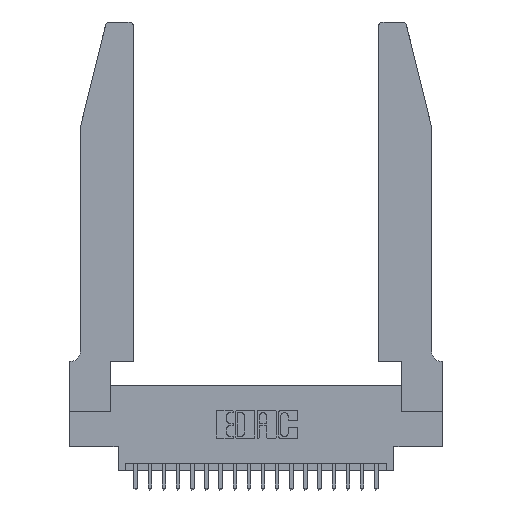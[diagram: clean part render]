
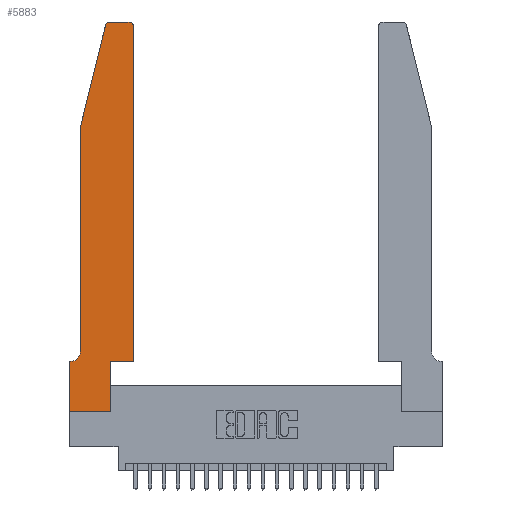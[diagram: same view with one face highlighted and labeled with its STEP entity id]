
A CAD part, top view. The second image highlights one B-rep face of the part: STEP entity #5883.
In plain terms, the highlighted planar face has unit normal (0, 0, 1).
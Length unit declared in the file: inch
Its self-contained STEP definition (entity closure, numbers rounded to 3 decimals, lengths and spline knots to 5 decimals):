
#41 = CARTESIAN_POINT ( 'NONE',  ( 0., 0., 0.37 ) ) ;
#44 = EDGE_CURVE ( 'NONE', #14610, #19202, #10375, .T. ) ;
#132 = AXIS2_PLACEMENT_3D ( 'NONE', #1566, #18614, #13588 ) ;
#656 = ORIENTED_EDGE ( 'NONE', *, *, #984, .T. ) ;
#933 = VERTEX_POINT ( 'NONE', #8329 ) ;
#984 = EDGE_CURVE ( 'NONE', #8225, #11975, #17523, .T. ) ;
#1009 = ORIENTED_EDGE ( 'NONE', *, *, #20802, .T. ) ;
#1018 = CARTESIAN_POINT ( 'NONE',  ( 0.4205, 2.72, 0.37 ) ) ;
#1566 = CARTESIAN_POINT ( 'NONE',  ( 0.0055, 0.42, 0.37 ) ) ;
#1724 = CARTESIAN_POINT ( 'NONE',  ( 0., 0.35, 0.37 ) ) ;
#2267 = CARTESIAN_POINT ( 'NONE',  ( 0.284, 2.72, 0.37 ) ) ;
#2514 = DIRECTION ( 'NONE',  ( 0., 1., 0. ) ) ;
#2550 = ORIENTED_EDGE ( 'NONE', *, *, #12534, .T. ) ;
#2740 = CARTESIAN_POINT ( 'NONE',  ( 0.2865, 0.35, 0.37 ) ) ;
#3406 = CARTESIAN_POINT ( 'NONE',  ( 0.4505, 0.35, 0.37 ) ) ;
#3928 = VERTEX_POINT ( 'NONE', #1724 ) ;
#4030 = DIRECTION ( 'NONE',  ( 0., 0., 1. ) ) ;
#4218 = FACE_OUTER_BOUND ( 'NONE', #7826, .T. ) ;
#4610 = EDGE_CURVE ( 'NONE', #16355, #19908, #15493, .T. ) ;
#4636 = CARTESIAN_POINT ( 'NONE',  ( 0.4505, 0.35, 0.37 ) ) ;
#4758 = CARTESIAN_POINT ( 'NONE',  ( 0.25487, 2.72718, 0.37 ) ) ;
#4825 = CARTESIAN_POINT ( 'NONE',  ( 0.4505, 2.72, 0.37 ) ) ;
#4875 = DIRECTION ( 'NONE',  ( -1., 0., 0. ) ) ;
#4888 = VECTOR ( 'NONE', #14288, 39.37008 ) ;
#5043 = LINE ( 'NONE', #41, #18176 ) ;
#5080 = VERTEX_POINT ( 'NONE', #9104 ) ;
#5250 = CARTESIAN_POINT ( 'NONE',  ( 0.0055, 0.35, 0.37 ) ) ;
#5457 = EDGE_CURVE ( 'NONE', #3928, #16355, #5043, .T. ) ;
#5693 = DIRECTION ( 'NONE',  ( 1., 0., 0. ) ) ;
#5883 = ADVANCED_FACE ( 'NONE', ( #4218 ), #20402, .T. ) ;
#5922 = LINE ( 'NONE', #2740, #9970 ) ;
#6152 = EDGE_CURVE ( 'NONE', #933, #8225, #17350, .T. ) ;
#6201 = DIRECTION ( 'NONE',  ( 0., 0., 1. ) ) ;
#6876 = CARTESIAN_POINT ( 'NONE',  ( 0.4205, 2.75, 0.37 ) ) ;
#6902 = CARTESIAN_POINT ( 'NONE',  ( 0., 0., 0.37 ) ) ;
#7506 = DIRECTION ( 'NONE',  ( 1., 0., 0. ) ) ;
#7527 = AXIS2_PLACEMENT_3D ( 'NONE', #1018, #6201, #19962 ) ;
#7616 = DIRECTION ( 'NONE',  ( -0.239, -0.971, 0. ) ) ;
#7826 = EDGE_LOOP ( 'NONE', ( #19796, #11047, #656, #20272, #12073, #1009, #19570, #15706, #2550, #9022, #21586, #9227 ) ) ;
#7940 = LINE ( 'NONE', #9996, #9011 ) ;
#8225 = VERTEX_POINT ( 'NONE', #4758 ) ;
#8329 = CARTESIAN_POINT ( 'NONE',  ( 0.284, 2.75, 0.37 ) ) ;
#8748 = DIRECTION ( 'NONE',  ( 1., 0., 0. ) ) ;
#9011 = VECTOR ( 'NONE', #4875, 39.37008 ) ;
#9022 = ORIENTED_EDGE ( 'NONE', *, *, #44, .T. ) ;
#9104 = CARTESIAN_POINT ( 'NONE',  ( 0.0755, 0.42, 0.37 ) ) ;
#9142 = CARTESIAN_POINT ( 'NONE',  ( 0.0755, 2., 0.37 ) ) ;
#9227 = ORIENTED_EDGE ( 'NONE', *, *, #13884, .T. ) ;
#9246 = AXIS2_PLACEMENT_3D ( 'NONE', #14853, #17541, #8748 ) ;
#9970 = VECTOR ( 'NONE', #2514, 39.37008 ) ;
#9996 = CARTESIAN_POINT ( 'NONE',  ( 0.0755, 0.35, 0.37 ) ) ;
#10375 = LINE ( 'NONE', #12525, #18400 ) ;
#10652 = LINE ( 'NONE', #18094, #14144 ) ;
#11047 = ORIENTED_EDGE ( 'NONE', *, *, #6152, .T. ) ;
#11252 = EDGE_CURVE ( 'NONE', #5080, #20966, #20241, .T. ) ;
#11975 = VERTEX_POINT ( 'NONE', #20164 ) ;
#12073 = ORIENTED_EDGE ( 'NONE', *, *, #11252, .T. ) ;
#12144 = LINE ( 'NONE', #9142, #4888 ) ;
#12525 = CARTESIAN_POINT ( 'NONE',  ( 0.4505, 0.35, 0.37 ) ) ;
#12534 = EDGE_CURVE ( 'NONE', #19908, #14610, #5922, .T. ) ;
#12634 = DIRECTION ( 'NONE',  ( 0., -1., 0. ) ) ;
#13588 = DIRECTION ( 'NONE',  ( -1., 0., 0. ) ) ;
#13836 = VERTEX_POINT ( 'NONE', #6876 ) ;
#13884 = EDGE_CURVE ( 'NONE', #20284, #13836, #17462, .T. ) ;
#14144 = VECTOR ( 'NONE', #21513, 39.37008 ) ;
#14288 = DIRECTION ( 'NONE',  ( 0., -1., 0. ) ) ;
#14610 = VERTEX_POINT ( 'NONE', #21944 ) ;
#14853 = CARTESIAN_POINT ( 'NONE',  ( 0., 0.35, 0.37 ) ) ;
#15485 = DIRECTION ( 'NONE',  ( 1., 0., 0. ) ) ;
#15493 = LINE ( 'NONE', #6902, #19824 ) ;
#15706 = ORIENTED_EDGE ( 'NONE', *, *, #4610, .T. ) ;
#16072 = EDGE_CURVE ( 'NONE', #13836, #933, #10652, .T. ) ;
#16355 = VERTEX_POINT ( 'NONE', #17452 ) ;
#16656 = EDGE_CURVE ( 'NONE', #19202, #20284, #20612, .T. ) ;
#16777 = DIRECTION ( 'NONE',  ( 0., 1., 0. ) ) ;
#17350 = CIRCLE ( 'NONE', #22041, 0.03 ) ;
#17452 = CARTESIAN_POINT ( 'NONE',  ( 0., 0., 0.37 ) ) ;
#17462 = CIRCLE ( 'NONE', #7527, 0.03 ) ;
#17523 = LINE ( 'NONE', #21414, #21873 ) ;
#17541 = DIRECTION ( 'NONE',  ( 0., 0., 1. ) ) ;
#17649 = CARTESIAN_POINT ( 'NONE',  ( 0.2865, 0., 0.37 ) ) ;
#18094 = CARTESIAN_POINT ( 'NONE',  ( 0.2605, 2.75, 0.37 ) ) ;
#18176 = VECTOR ( 'NONE', #12634, 39.37008 ) ;
#18400 = VECTOR ( 'NONE', #5693, 39.37008 ) ;
#18614 = DIRECTION ( 'NONE',  ( 0., 0., -1. ) ) ;
#19202 = VERTEX_POINT ( 'NONE', #3406 ) ;
#19393 = EDGE_CURVE ( 'NONE', #11975, #5080, #12144, .T. ) ;
#19570 = ORIENTED_EDGE ( 'NONE', *, *, #5457, .T. ) ;
#19796 = ORIENTED_EDGE ( 'NONE', *, *, #16072, .T. ) ;
#19824 = VECTOR ( 'NONE', #15485, 39.37008 ) ;
#19908 = VERTEX_POINT ( 'NONE', #17649 ) ;
#19962 = DIRECTION ( 'NONE',  ( 1., 0., 0. ) ) ;
#20044 = VECTOR ( 'NONE', #16777, 39.37008 ) ;
#20164 = CARTESIAN_POINT ( 'NONE',  ( 0.0755, 2., 0.37 ) ) ;
#20241 = CIRCLE ( 'NONE', #132, 0.07 ) ;
#20272 = ORIENTED_EDGE ( 'NONE', *, *, #19393, .T. ) ;
#20284 = VERTEX_POINT ( 'NONE', #4825 ) ;
#20402 = PLANE ( 'NONE',  #9246 ) ;
#20612 = LINE ( 'NONE', #4636, #20044 ) ;
#20802 = EDGE_CURVE ( 'NONE', #20966, #3928, #7940, .T. ) ;
#20966 = VERTEX_POINT ( 'NONE', #5250 ) ;
#21414 = CARTESIAN_POINT ( 'NONE',  ( 0.0755, 2., 0.37 ) ) ;
#21513 = DIRECTION ( 'NONE',  ( -1., 0., 0. ) ) ;
#21586 = ORIENTED_EDGE ( 'NONE', *, *, #16656, .T. ) ;
#21873 = VECTOR ( 'NONE', #7616, 39.37008 ) ;
#21944 = CARTESIAN_POINT ( 'NONE',  ( 0.2865, 0.35, 0.37 ) ) ;
#22041 = AXIS2_PLACEMENT_3D ( 'NONE', #2267, #4030, #7506 ) ;
